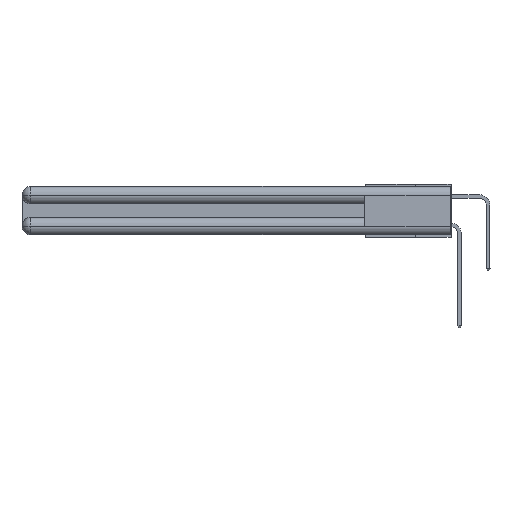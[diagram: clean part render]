
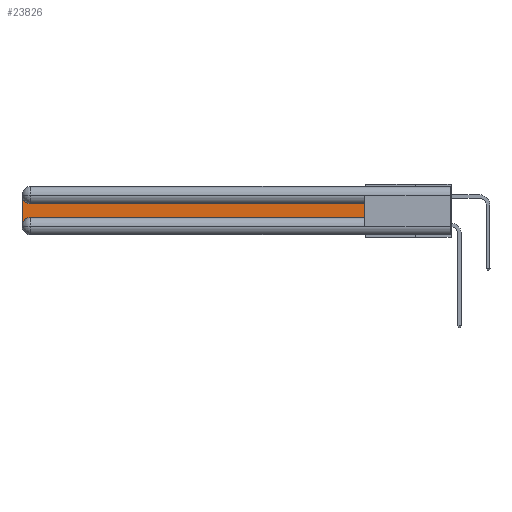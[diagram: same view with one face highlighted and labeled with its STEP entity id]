
A CAD part, left-side view. The second image highlights one B-rep face of the part: STEP entity #23826.
In plain terms, the highlighted planar face has unit normal (-1, 0, 0).
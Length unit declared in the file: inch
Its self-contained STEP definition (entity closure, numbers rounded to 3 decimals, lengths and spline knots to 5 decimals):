
#279 = DIRECTION ( 'NONE',  ( 0., 0., -1. ) ) ;
#315 = VECTOR ( 'NONE', #8827, 39.37008 ) ;
#342 = CARTESIAN_POINT ( 'NONE',  ( 0.075, 2.94, -0.0625 ) ) ;
#556 = VERTEX_POINT ( 'NONE', #577 ) ;
#577 = CARTESIAN_POINT ( 'NONE',  ( 0.075, 3., -0.2775 ) ) ;
#981 = VERTEX_POINT ( 'NONE', #23623 ) ;
#1339 = EDGE_CURVE ( 'NONE', #22443, #14469, #24807, .T. ) ;
#2058 = AXIS2_PLACEMENT_3D ( 'NONE', #19655, #23980, #279 ) ;
#2304 = CARTESIAN_POINT ( 'NONE',  ( 0.075, 0.6, -0.1225 ) ) ;
#2459 = DIRECTION ( 'NONE',  ( 0., 0., -1. ) ) ;
#3642 = EDGE_CURVE ( 'NONE', #556, #22443, #24833, .T. ) ;
#4386 = EDGE_CURVE ( 'NONE', #14469, #11695, #26144, .T. ) ;
#5347 = LINE ( 'NONE', #6063, #18896 ) ;
#5543 = AXIS2_PLACEMENT_3D ( 'NONE', #8339, #12707, #25722 ) ;
#6063 = CARTESIAN_POINT ( 'NONE',  ( 0.075, 3., -0.2175 ) ) ;
#7486 = ORIENTED_EDGE ( 'NONE', *, *, #20786, .T. ) ;
#7755 = DIRECTION ( 'NONE',  ( 0., -1., 0. ) ) ;
#8236 = VECTOR ( 'NONE', #12769, 39.37008 ) ;
#8302 = CARTESIAN_POINT ( 'NONE',  ( 0.075, 2.94, -0.2175 ) ) ;
#8339 = CARTESIAN_POINT ( 'NONE',  ( 0.075, 3., -0.1225 ) ) ;
#8827 = DIRECTION ( 'NONE',  ( 0., 1., 0. ) ) ;
#10307 = CIRCLE ( 'NONE', #17299, 0.06 ) ;
#11695 = VERTEX_POINT ( 'NONE', #12491 ) ;
#12491 = CARTESIAN_POINT ( 'NONE',  ( 0.075, 0.6, -0.1225 ) ) ;
#12666 = VECTOR ( 'NONE', #7755, 39.37008 ) ;
#12707 = DIRECTION ( 'NONE',  ( 1., 0., 0. ) ) ;
#12769 = DIRECTION ( 'NONE',  ( 0., 0., 1. ) ) ;
#13896 = CARTESIAN_POINT ( 'NONE',  ( 0.075, 0.6, -0.2175 ) ) ;
#14011 = DIRECTION ( 'NONE',  ( 0., 0., -1. ) ) ;
#14469 = VERTEX_POINT ( 'NONE', #17521 ) ;
#14996 = VERTEX_POINT ( 'NONE', #27805 ) ;
#16887 = LINE ( 'NONE', #2304, #315 ) ;
#17299 = AXIS2_PLACEMENT_3D ( 'NONE', #342, #24432, #14011 ) ;
#17310 = PLANE ( 'NONE',  #5543 ) ;
#17521 = CARTESIAN_POINT ( 'NONE',  ( 0.075, 0.6, -0.2175 ) ) ;
#18727 = FACE_OUTER_BOUND ( 'NONE', #25230, .T. ) ;
#18896 = VECTOR ( 'NONE', #2459, 39.37008 ) ;
#19655 = CARTESIAN_POINT ( 'NONE',  ( 0.075, 2.94, -0.2775 ) ) ;
#20336 = EDGE_CURVE ( 'NONE', #11695, #14996, #16887, .T. ) ;
#20606 = CARTESIAN_POINT ( 'NONE',  ( 0.075, 0.6, -0.2175 ) ) ;
#20786 = EDGE_CURVE ( 'NONE', #981, #556, #5347, .T. ) ;
#22443 = VERTEX_POINT ( 'NONE', #8302 ) ;
#23059 = EDGE_CURVE ( 'NONE', #14996, #981, #10307, .T. ) ;
#23350 = ORIENTED_EDGE ( 'NONE', *, *, #4386, .T. ) ;
#23623 = CARTESIAN_POINT ( 'NONE',  ( 0.075, 3., -0.0625 ) ) ;
#23826 = ADVANCED_FACE ( 'NONE', ( #18727 ), #17310, .F. ) ;
#23980 = DIRECTION ( 'NONE',  ( 1., 0., 0. ) ) ;
#24432 = DIRECTION ( 'NONE',  ( 1., 0., 0. ) ) ;
#24488 = ORIENTED_EDGE ( 'NONE', *, *, #23059, .T. ) ;
#24807 = LINE ( 'NONE', #13896, #12666 ) ;
#24833 = CIRCLE ( 'NONE', #2058, 0.06 ) ;
#25230 = EDGE_LOOP ( 'NONE', ( #25625, #24488, #7486, #26871, #27970, #23350 ) ) ;
#25625 = ORIENTED_EDGE ( 'NONE', *, *, #20336, .T. ) ;
#25722 = DIRECTION ( 'NONE',  ( 0., 0., -1. ) ) ;
#26144 = LINE ( 'NONE', #20606, #8236 ) ;
#26871 = ORIENTED_EDGE ( 'NONE', *, *, #3642, .T. ) ;
#27805 = CARTESIAN_POINT ( 'NONE',  ( 0.075, 2.94, -0.1225 ) ) ;
#27970 = ORIENTED_EDGE ( 'NONE', *, *, #1339, .T. ) ;
